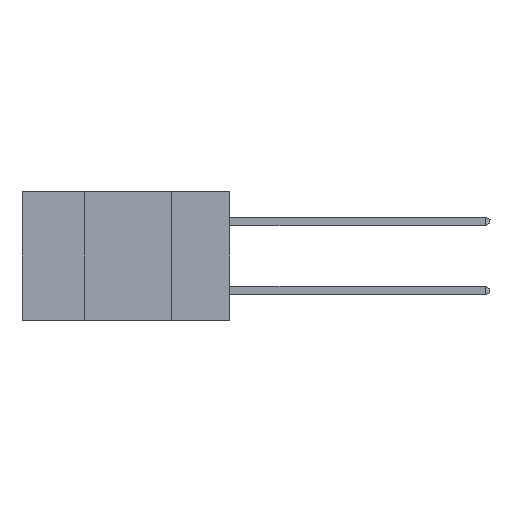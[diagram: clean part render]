
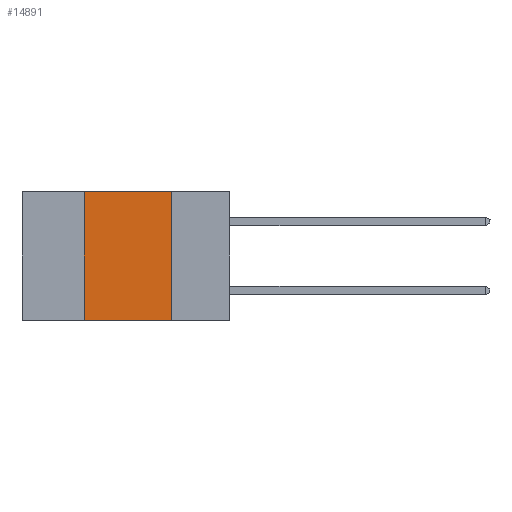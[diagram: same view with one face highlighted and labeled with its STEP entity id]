
A CAD part, left-side view. The second image highlights one B-rep face of the part: STEP entity #14891.
In plain terms, the highlighted planar face has unit normal (-1, 0, 0).
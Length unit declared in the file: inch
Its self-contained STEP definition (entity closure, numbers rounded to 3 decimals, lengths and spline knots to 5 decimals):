
#889 = EDGE_CURVE ( 'NONE', #13475, #7308, #16660, .T. ) ;
#1255 = DIRECTION ( 'NONE',  ( 0., -1., 0. ) ) ;
#1642 = EDGE_CURVE ( 'NONE', #16436, #13475, #21708, .T. ) ;
#2654 = DIRECTION ( 'NONE',  ( 0., -1., 0. ) ) ;
#3355 = CARTESIAN_POINT ( 'NONE',  ( 0., 0.42, 0. ) ) ;
#4608 = AXIS2_PLACEMENT_3D ( 'NONE', #21663, #4852, #21763 ) ;
#4852 = DIRECTION ( 'NONE',  ( 1., 0., 0. ) ) ;
#5059 = CARTESIAN_POINT ( 'NONE',  ( 0., 0.17, -0.37 ) ) ;
#5308 = VECTOR ( 'NONE', #2654, 39.37008 ) ;
#6969 = EDGE_CURVE ( 'NONE', #10574, #7308, #10944, .T. ) ;
#7014 = CARTESIAN_POINT ( 'NONE',  ( 0., 0.17, 0. ) ) ;
#7308 = VERTEX_POINT ( 'NONE', #15552 ) ;
#7957 = ORIENTED_EDGE ( 'NONE', *, *, #20922, .F. ) ;
#10020 = PLANE ( 'NONE',  #4608 ) ;
#10574 = VERTEX_POINT ( 'NONE', #16003 ) ;
#10777 = ORIENTED_EDGE ( 'NONE', *, *, #889, .F. ) ;
#10944 = LINE ( 'NONE', #12910, #5308 ) ;
#11039 = LINE ( 'NONE', #15913, #16478 ) ;
#11479 = ORIENTED_EDGE ( 'NONE', *, *, #6969, .T. ) ;
#11660 = VECTOR ( 'NONE', #1255, 39.37008 ) ;
#12818 = VECTOR ( 'NONE', #19869, 39.37008 ) ;
#12910 = CARTESIAN_POINT ( 'NONE',  ( 0., 0.6, -0.37 ) ) ;
#13475 = VERTEX_POINT ( 'NONE', #7014 ) ;
#14882 = FACE_OUTER_BOUND ( 'NONE', #16054, .T. ) ;
#14891 = ADVANCED_FACE ( 'NONE', ( #14882 ), #10020, .F. ) ;
#15028 = CARTESIAN_POINT ( 'NONE',  ( 0., 0.6, 0. ) ) ;
#15552 = CARTESIAN_POINT ( 'NONE',  ( 0., 0.17, -0.37 ) ) ;
#15788 = DIRECTION ( 'NONE',  ( 0., 0., 1. ) ) ;
#15913 = CARTESIAN_POINT ( 'NONE',  ( 0., 0.42, -0.37 ) ) ;
#16003 = CARTESIAN_POINT ( 'NONE',  ( 0., 0.42, -0.37 ) ) ;
#16054 = EDGE_LOOP ( 'NONE', ( #10777, #21313, #7957, #11479 ) ) ;
#16436 = VERTEX_POINT ( 'NONE', #3355 ) ;
#16478 = VECTOR ( 'NONE', #15788, 39.37008 ) ;
#16660 = LINE ( 'NONE', #5059, #12818 ) ;
#19869 = DIRECTION ( 'NONE',  ( 0., 0., -1. ) ) ;
#20922 = EDGE_CURVE ( 'NONE', #10574, #16436, #11039, .T. ) ;
#21313 = ORIENTED_EDGE ( 'NONE', *, *, #1642, .F. ) ;
#21663 = CARTESIAN_POINT ( 'NONE',  ( 0., 0.6, 0. ) ) ;
#21708 = LINE ( 'NONE', #15028, #11660 ) ;
#21763 = DIRECTION ( 'NONE',  ( 0., 0., -1. ) ) ;
